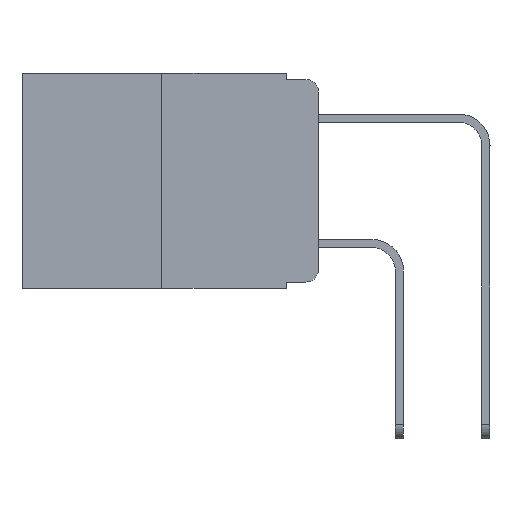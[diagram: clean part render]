
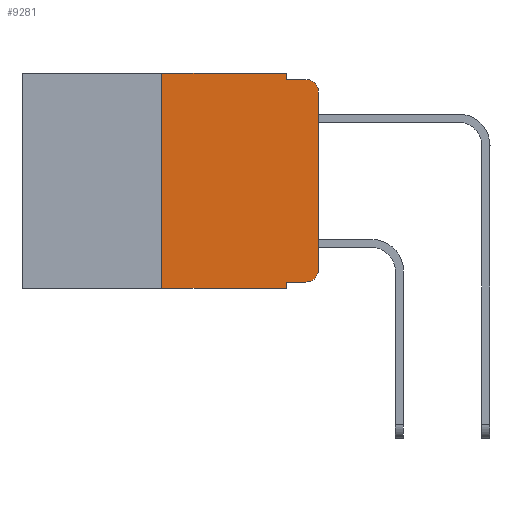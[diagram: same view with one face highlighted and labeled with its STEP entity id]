
A CAD part, left-side view. The second image highlights one B-rep face of the part: STEP entity #9281.
In plain terms, the highlighted planar face has unit normal (-1, 0, 0).
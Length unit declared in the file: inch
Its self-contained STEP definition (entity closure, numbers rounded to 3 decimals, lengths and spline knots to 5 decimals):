
#39 = CARTESIAN_POINT ( 'NONE',  ( 0., 0.051, -0.01 ) ) ;
#111 = ORIENTED_EDGE ( 'NONE', *, *, #4331, .T. ) ;
#255 = VERTEX_POINT ( 'NONE', #13053 ) ;
#258 = ORIENTED_EDGE ( 'NONE', *, *, #7058, .T. ) ;
#683 = LINE ( 'NONE', #10514, #1217 ) ;
#755 = EDGE_CURVE ( 'NONE', #13518, #2903, #13227, .T. ) ;
#1092 = LINE ( 'NONE', #7753, #6445 ) ;
#1217 = VECTOR ( 'NONE', #11654, 39.37008 ) ;
#1224 = VERTEX_POINT ( 'NONE', #14094 ) ;
#1471 = FACE_OUTER_BOUND ( 'NONE', #7469, .T. ) ;
#1684 = CARTESIAN_POINT ( 'NONE',  ( 0., 0.473, -0.343 ) ) ;
#1783 = CARTESIAN_POINT ( 'NONE',  ( 0., 0.051, -0.343 ) ) ;
#1899 = CIRCLE ( 'NONE', #7767, 0.02 ) ;
#2005 = ORIENTED_EDGE ( 'NONE', *, *, #10472, .F. ) ;
#2098 = VERTEX_POINT ( 'NONE', #12969 ) ;
#2305 = CARTESIAN_POINT ( 'NONE',  ( 0., 0.051, -0.333 ) ) ;
#2404 = LINE ( 'NONE', #14236, #5235 ) ;
#2434 = ORIENTED_EDGE ( 'NONE', *, *, #14093, .T. ) ;
#2903 = VERTEX_POINT ( 'NONE', #8575 ) ;
#2969 = VERTEX_POINT ( 'NONE', #9715 ) ;
#3202 = DIRECTION ( 'NONE',  ( -1., 0., 0. ) ) ;
#3426 = ORIENTED_EDGE ( 'NONE', *, *, #6236, .F. ) ;
#4331 = EDGE_CURVE ( 'NONE', #13035, #255, #683, .T. ) ;
#4360 = CARTESIAN_POINT ( 'NONE',  ( 0., 0.473, 0. ) ) ;
#4491 = ORIENTED_EDGE ( 'NONE', *, *, #755, .F. ) ;
#5231 = LINE ( 'NONE', #14575, #8620 ) ;
#5235 = VECTOR ( 'NONE', #11811, 39.37008 ) ;
#5334 = VERTEX_POINT ( 'NONE', #5725 ) ;
#5426 = CARTESIAN_POINT ( 'NONE',  ( 0., 0.25, -0.343 ) ) ;
#5466 = CARTESIAN_POINT ( 'NONE',  ( 0., 0., 0. ) ) ;
#5555 = DIRECTION ( 'NONE',  ( 1., 0., 0. ) ) ;
#5593 = DIRECTION ( 'NONE',  ( 0., 0., -1. ) ) ;
#5647 = EDGE_CURVE ( 'NONE', #11286, #1224, #1899, .T. ) ;
#5725 = CARTESIAN_POINT ( 'NONE',  ( 0., 0.051, -0.01 ) ) ;
#6236 = EDGE_CURVE ( 'NONE', #13035, #9777, #2404, .T. ) ;
#6445 = VECTOR ( 'NONE', #6517, 39.37008 ) ;
#6517 = DIRECTION ( 'NONE',  ( 0., 0., -1. ) ) ;
#6648 = DIRECTION ( 'NONE',  ( 0., 0., 1. ) ) ;
#6937 = CARTESIAN_POINT ( 'NONE',  ( 0., 0., -0.03 ) ) ;
#7058 = EDGE_CURVE ( 'NONE', #13518, #9777, #13613, .T. ) ;
#7469 = EDGE_LOOP ( 'NONE', ( #2434, #7765, #14382, #2005, #10162, #4491, #258, #3426, #111, #9694 ) ) ;
#7525 = LINE ( 'NONE', #39, #7699 ) ;
#7529 = DIRECTION ( 'NONE',  ( 0., 0., -1. ) ) ;
#7674 = AXIS2_PLACEMENT_3D ( 'NONE', #14579, #3202, #13486 ) ;
#7699 = VECTOR ( 'NONE', #9219, 39.37008 ) ;
#7753 = CARTESIAN_POINT ( 'NONE',  ( 0., 0.051, 0. ) ) ;
#7765 = ORIENTED_EDGE ( 'NONE', *, *, #5647, .T. ) ;
#7767 = AXIS2_PLACEMENT_3D ( 'NONE', #13257, #8597, #7529 ) ;
#7970 = EDGE_CURVE ( 'NONE', #2903, #2098, #5231, .T. ) ;
#8122 = DIRECTION ( 'NONE',  ( 0., 0., 1. ) ) ;
#8575 = CARTESIAN_POINT ( 'NONE',  ( 0., 0.25, 0. ) ) ;
#8597 = DIRECTION ( 'NONE',  ( -1., 0., 0. ) ) ;
#8620 = VECTOR ( 'NONE', #10315, 39.37008 ) ;
#8993 = VECTOR ( 'NONE', #13068, 39.37008 ) ;
#9203 = CIRCLE ( 'NONE', #7674, 0.02 ) ;
#9219 = DIRECTION ( 'NONE',  ( 0., -1., 0. ) ) ;
#9281 = ADVANCED_FACE ( 'NONE', ( #1471 ), #12360, .F. ) ;
#9448 = CARTESIAN_POINT ( 'NONE',  ( 0., 0.25, 0. ) ) ;
#9694 = ORIENTED_EDGE ( 'NONE', *, *, #12338, .T. ) ;
#9715 = CARTESIAN_POINT ( 'NONE',  ( 0., 0., -0.313 ) ) ;
#9777 = VERTEX_POINT ( 'NONE', #1783 ) ;
#10041 = EDGE_CURVE ( 'NONE', #5334, #1224, #7525, .T. ) ;
#10162 = ORIENTED_EDGE ( 'NONE', *, *, #7970, .F. ) ;
#10315 = DIRECTION ( 'NONE',  ( 0., -1., 0. ) ) ;
#10437 = AXIS2_PLACEMENT_3D ( 'NONE', #4360, #5555, #5593 ) ;
#10472 = EDGE_CURVE ( 'NONE', #2098, #5334, #1092, .T. ) ;
#10514 = CARTESIAN_POINT ( 'NONE',  ( 0., 0.051, -0.333 ) ) ;
#10532 = LINE ( 'NONE', #5466, #11971 ) ;
#11286 = VERTEX_POINT ( 'NONE', #6937 ) ;
#11654 = DIRECTION ( 'NONE',  ( 0., -1., 0. ) ) ;
#11811 = DIRECTION ( 'NONE',  ( 0., 0., -1. ) ) ;
#11971 = VECTOR ( 'NONE', #6648, 39.37008 ) ;
#12338 = EDGE_CURVE ( 'NONE', #255, #2969, #9203, .T. ) ;
#12360 = PLANE ( 'NONE',  #10437 ) ;
#12969 = CARTESIAN_POINT ( 'NONE',  ( 0., 0.051, 0. ) ) ;
#13035 = VERTEX_POINT ( 'NONE', #2305 ) ;
#13044 = VECTOR ( 'NONE', #8122, 39.37008 ) ;
#13053 = CARTESIAN_POINT ( 'NONE',  ( 0., 0.02, -0.333 ) ) ;
#13068 = DIRECTION ( 'NONE',  ( 0., -1., 0. ) ) ;
#13227 = LINE ( 'NONE', #9448, #13044 ) ;
#13257 = CARTESIAN_POINT ( 'NONE',  ( 0., 0.02, -0.03 ) ) ;
#13486 = DIRECTION ( 'NONE',  ( 0., 0., -1. ) ) ;
#13518 = VERTEX_POINT ( 'NONE', #5426 ) ;
#13613 = LINE ( 'NONE', #1684, #8993 ) ;
#14093 = EDGE_CURVE ( 'NONE', #2969, #11286, #10532, .T. ) ;
#14094 = CARTESIAN_POINT ( 'NONE',  ( 0., 0.02, -0.01 ) ) ;
#14236 = CARTESIAN_POINT ( 'NONE',  ( 0., 0.051, 0. ) ) ;
#14382 = ORIENTED_EDGE ( 'NONE', *, *, #10041, .F. ) ;
#14575 = CARTESIAN_POINT ( 'NONE',  ( 0., 0.473, 0. ) ) ;
#14579 = CARTESIAN_POINT ( 'NONE',  ( 0., 0.02, -0.313 ) ) ;
